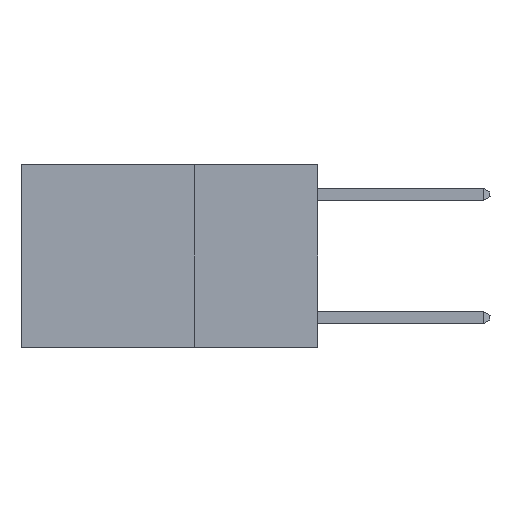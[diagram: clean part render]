
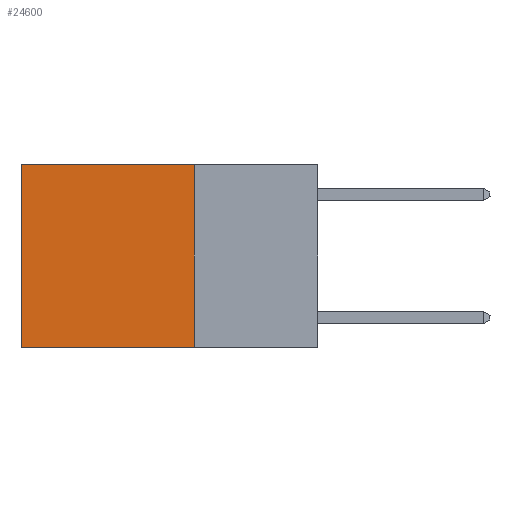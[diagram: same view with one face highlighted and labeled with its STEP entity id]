
A CAD part, left-side view. The second image highlights one B-rep face of the part: STEP entity #24600.
In plain terms, the highlighted planar face has unit normal (-1, 0, 0).
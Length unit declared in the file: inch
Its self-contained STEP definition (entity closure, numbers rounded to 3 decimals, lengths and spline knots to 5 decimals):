
#420 = CARTESIAN_POINT ( 'NONE',  ( 0.2625, 0.25, 0. ) ) ;
#1131 = VECTOR ( 'NONE', #7567, 39.37008 ) ;
#1167 = LINE ( 'NONE', #29898, #29464 ) ;
#2723 = VECTOR ( 'NONE', #25470, 39.37008 ) ;
#3196 = EDGE_CURVE ( 'NONE', #14510, #30824, #7891, .T. ) ;
#3953 = ORIENTED_EDGE ( 'NONE', *, *, #4222, .F. ) ;
#4222 = EDGE_CURVE ( 'NONE', #10764, #20969, #1167, .T. ) ;
#4726 = CARTESIAN_POINT ( 'NONE',  ( 0.2625, 0.25, -0.37 ) ) ;
#6006 = DIRECTION ( 'NONE',  ( 0., 0., -1. ) ) ;
#7477 = DIRECTION ( 'NONE',  ( 1., 0., 0. ) ) ;
#7558 = ORIENTED_EDGE ( 'NONE', *, *, #24396, .F. ) ;
#7567 = DIRECTION ( 'NONE',  ( 0., 1., 0. ) ) ;
#7891 = LINE ( 'NONE', #14962, #1131 ) ;
#8675 = CARTESIAN_POINT ( 'NONE',  ( 0.2625, 0.6, 0. ) ) ;
#8803 = AXIS2_PLACEMENT_3D ( 'NONE', #17973, #7477, #6006 ) ;
#9795 = ORIENTED_EDGE ( 'NONE', *, *, #23544, .T. ) ;
#10764 = VERTEX_POINT ( 'NONE', #4726 ) ;
#11020 = EDGE_LOOP ( 'NONE', ( #9795, #3953, #7558, #21111 ) ) ;
#13476 = DIRECTION ( 'NONE',  ( 0., 0., -1. ) ) ;
#14510 = VERTEX_POINT ( 'NONE', #420 ) ;
#14962 = CARTESIAN_POINT ( 'NONE',  ( 0.2625, 0.25, 0. ) ) ;
#17973 = CARTESIAN_POINT ( 'NONE',  ( 0.2625, 0.25, 0. ) ) ;
#18213 = CARTESIAN_POINT ( 'NONE',  ( 0.2625, 0.6, 0. ) ) ;
#20183 = DIRECTION ( 'NONE',  ( 0., 1., 0. ) ) ;
#20615 = LINE ( 'NONE', #8675, #2723 ) ;
#20969 = VERTEX_POINT ( 'NONE', #30266 ) ;
#21111 = ORIENTED_EDGE ( 'NONE', *, *, #3196, .T. ) ;
#23544 = EDGE_CURVE ( 'NONE', #30824, #20969, #20615, .T. ) ;
#23838 = VECTOR ( 'NONE', #13476, 39.37008 ) ;
#24396 = EDGE_CURVE ( 'NONE', #14510, #10764, #27437, .T. ) ;
#24600 = ADVANCED_FACE ( 'NONE', ( #27514 ), #27362, .F. ) ;
#25470 = DIRECTION ( 'NONE',  ( 0., 0., -1. ) ) ;
#27362 = PLANE ( 'NONE',  #8803 ) ;
#27437 = LINE ( 'NONE', #29941, #23838 ) ;
#27514 = FACE_OUTER_BOUND ( 'NONE', #11020, .T. ) ;
#29464 = VECTOR ( 'NONE', #20183, 39.37008 ) ;
#29898 = CARTESIAN_POINT ( 'NONE',  ( 0.2625, 0.25, -0.37 ) ) ;
#29941 = CARTESIAN_POINT ( 'NONE',  ( 0.2625, 0.25, 0. ) ) ;
#30266 = CARTESIAN_POINT ( 'NONE',  ( 0.2625, 0.6, -0.37 ) ) ;
#30824 = VERTEX_POINT ( 'NONE', #18213 ) ;
